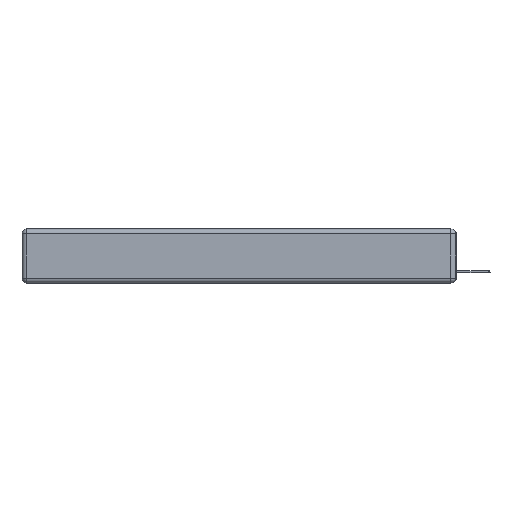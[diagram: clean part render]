
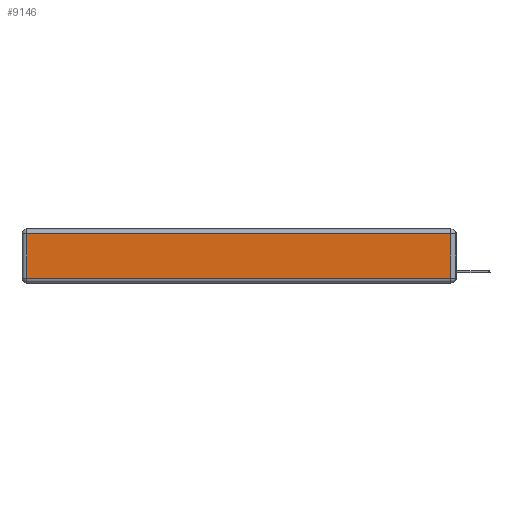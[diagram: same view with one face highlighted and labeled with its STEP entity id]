
A CAD part, left-side view. The second image highlights one B-rep face of the part: STEP entity #9146.
In plain terms, the highlighted planar face has unit normal (-1, 0, 0).
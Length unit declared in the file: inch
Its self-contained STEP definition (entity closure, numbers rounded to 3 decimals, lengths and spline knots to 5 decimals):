
#57 = CARTESIAN_POINT ( 'NONE',  ( 0., 0., -0.343 ) ) ;
#139 = EDGE_CURVE ( 'NONE', #2912, #9877, #4058, .T. ) ;
#927 = DIRECTION ( 'NONE',  ( 0., 1., 0. ) ) ;
#1171 = EDGE_CURVE ( 'NONE', #9877, #1477, #4926, .T. ) ;
#1275 = CARTESIAN_POINT ( 'NONE',  ( 0., 0.03, -0.343 ) ) ;
#1477 = VERTEX_POINT ( 'NONE', #4277 ) ;
#1651 = ORIENTED_EDGE ( 'NONE', *, *, #7510, .T. ) ;
#1759 = PLANE ( 'NONE',  #4596 ) ;
#2291 = CARTESIAN_POINT ( 'NONE',  ( 0., 2.72, -0.313 ) ) ;
#2912 = VERTEX_POINT ( 'NONE', #9053 ) ;
#3201 = ORIENTED_EDGE ( 'NONE', *, *, #139, .T. ) ;
#4012 = ORIENTED_EDGE ( 'NONE', *, *, #4961, .T. ) ;
#4058 = LINE ( 'NONE', #1275, #8394 ) ;
#4179 = DIRECTION ( 'NONE',  ( 0., 0., 1. ) ) ;
#4193 = CARTESIAN_POINT ( 'NONE',  ( 0., 0., -0.313 ) ) ;
#4277 = CARTESIAN_POINT ( 'NONE',  ( 0., 2.72, -0.03 ) ) ;
#4596 = AXIS2_PLACEMENT_3D ( 'NONE', #57, #10422, #6671 ) ;
#4671 = FACE_OUTER_BOUND ( 'NONE', #7503, .T. ) ;
#4926 = LINE ( 'NONE', #7491, #9417 ) ;
#4961 = EDGE_CURVE ( 'NONE', #11212, #2912, #10646, .T. ) ;
#5203 = ORIENTED_EDGE ( 'NONE', *, *, #1171, .T. ) ;
#6502 = VECTOR ( 'NONE', #10941, 39.37008 ) ;
#6671 = DIRECTION ( 'NONE',  ( 0., 0., 1. ) ) ;
#7491 = CARTESIAN_POINT ( 'NONE',  ( 0., 2.75, -0.03 ) ) ;
#7503 = EDGE_LOOP ( 'NONE', ( #4012, #3201, #5203, #1651 ) ) ;
#7510 = EDGE_CURVE ( 'NONE', #1477, #11212, #9032, .T. ) ;
#7942 = DIRECTION ( 'NONE',  ( 0., -1., 0. ) ) ;
#8394 = VECTOR ( 'NONE', #4179, 39.37008 ) ;
#9032 = LINE ( 'NONE', #9878, #6502 ) ;
#9053 = CARTESIAN_POINT ( 'NONE',  ( 0., 0.03, -0.313 ) ) ;
#9146 = ADVANCED_FACE ( 'NONE', ( #4671 ), #1759, .T. ) ;
#9417 = VECTOR ( 'NONE', #927, 39.37008 ) ;
#9877 = VERTEX_POINT ( 'NONE', #11526 ) ;
#9878 = CARTESIAN_POINT ( 'NONE',  ( 0., 2.72, -0.343 ) ) ;
#10422 = DIRECTION ( 'NONE',  ( -1., 0., 0. ) ) ;
#10499 = VECTOR ( 'NONE', #7942, 39.37008 ) ;
#10646 = LINE ( 'NONE', #4193, #10499 ) ;
#10941 = DIRECTION ( 'NONE',  ( 0., 0., -1. ) ) ;
#11212 = VERTEX_POINT ( 'NONE', #2291 ) ;
#11526 = CARTESIAN_POINT ( 'NONE',  ( 0., 0.03, -0.03 ) ) ;
